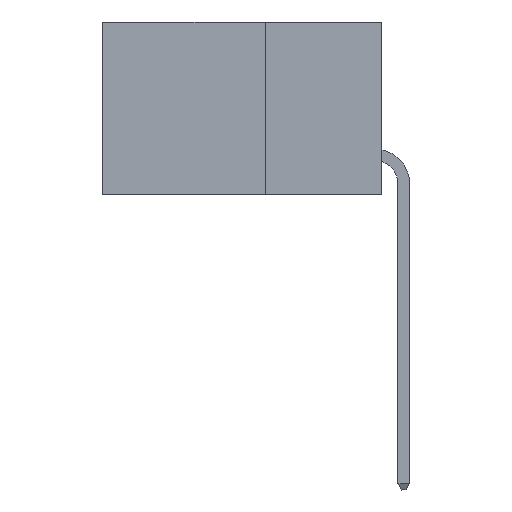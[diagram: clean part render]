
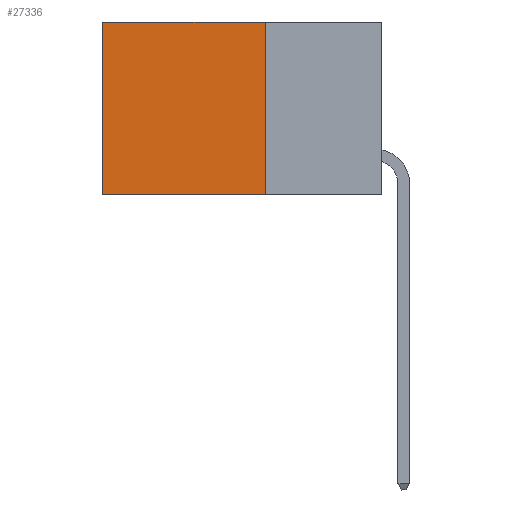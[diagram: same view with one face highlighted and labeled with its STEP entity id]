
A CAD part, left-side view. The second image highlights one B-rep face of the part: STEP entity #27336.
In plain terms, the highlighted planar face has unit normal (-1, 0, 0).
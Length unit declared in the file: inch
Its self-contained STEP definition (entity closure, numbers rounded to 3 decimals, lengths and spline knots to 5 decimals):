
#2566 = CARTESIAN_POINT ( 'NONE',  ( 0.2875, 0.6, 0. ) ) ;
#3022 = EDGE_CURVE ( 'NONE', #23112, #5040, #12490, .T. ) ;
#5040 = VERTEX_POINT ( 'NONE', #31717 ) ;
#5423 = DIRECTION ( 'NONE',  ( 1., 0., 0. ) ) ;
#5717 = VECTOR ( 'NONE', #7790, 39.37008 ) ;
#7790 = DIRECTION ( 'NONE',  ( 0., 0., -1. ) ) ;
#8624 = LINE ( 'NONE', #15686, #21247 ) ;
#9590 = CARTESIAN_POINT ( 'NONE',  ( 0.2875, 0.25, 0. ) ) ;
#10468 = PLANE ( 'NONE',  #13992 ) ;
#10726 = DIRECTION ( 'NONE',  ( 0., 1., 0. ) ) ;
#12191 = VERTEX_POINT ( 'NONE', #23630 ) ;
#12490 = LINE ( 'NONE', #2566, #5717 ) ;
#13992 = AXIS2_PLACEMENT_3D ( 'NONE', #28162, #5423, #23162 ) ;
#14861 = ORIENTED_EDGE ( 'NONE', *, *, #19554, .F. ) ;
#15138 = DIRECTION ( 'NONE',  ( 0., 0., -1. ) ) ;
#15686 = CARTESIAN_POINT ( 'NONE',  ( 0.2875, 0.25, 0. ) ) ;
#16375 = LINE ( 'NONE', #23377, #29052 ) ;
#16812 = CARTESIAN_POINT ( 'NONE',  ( 0.2875, 0.6, 0. ) ) ;
#18638 = EDGE_CURVE ( 'NONE', #12191, #5040, #16375, .T. ) ;
#19554 = EDGE_CURVE ( 'NONE', #24351, #12191, #21466, .T. ) ;
#21247 = VECTOR ( 'NONE', #10726, 39.37008 ) ;
#21466 = LINE ( 'NONE', #27765, #27409 ) ;
#23112 = VERTEX_POINT ( 'NONE', #16812 ) ;
#23162 = DIRECTION ( 'NONE',  ( 0., 0., -1. ) ) ;
#23377 = CARTESIAN_POINT ( 'NONE',  ( 0.2875, 0.25, -0.37 ) ) ;
#23630 = CARTESIAN_POINT ( 'NONE',  ( 0.2875, 0.25, -0.37 ) ) ;
#24351 = VERTEX_POINT ( 'NONE', #9590 ) ;
#25936 = DIRECTION ( 'NONE',  ( 0., 1., 0. ) ) ;
#27177 = ORIENTED_EDGE ( 'NONE', *, *, #18638, .F. ) ;
#27336 = ADVANCED_FACE ( 'NONE', ( #31167 ), #10468, .F. ) ;
#27409 = VECTOR ( 'NONE', #15138, 39.37008 ) ;
#27765 = CARTESIAN_POINT ( 'NONE',  ( 0.2875, 0.25, 0. ) ) ;
#28162 = CARTESIAN_POINT ( 'NONE',  ( 0.2875, 0.25, 0. ) ) ;
#28206 = EDGE_LOOP ( 'NONE', ( #29644, #27177, #14861, #31468 ) ) ;
#29052 = VECTOR ( 'NONE', #25936, 39.37008 ) ;
#29644 = ORIENTED_EDGE ( 'NONE', *, *, #3022, .T. ) ;
#30098 = EDGE_CURVE ( 'NONE', #24351, #23112, #8624, .T. ) ;
#31167 = FACE_OUTER_BOUND ( 'NONE', #28206, .T. ) ;
#31468 = ORIENTED_EDGE ( 'NONE', *, *, #30098, .T. ) ;
#31717 = CARTESIAN_POINT ( 'NONE',  ( 0.2875, 0.6, -0.37 ) ) ;
